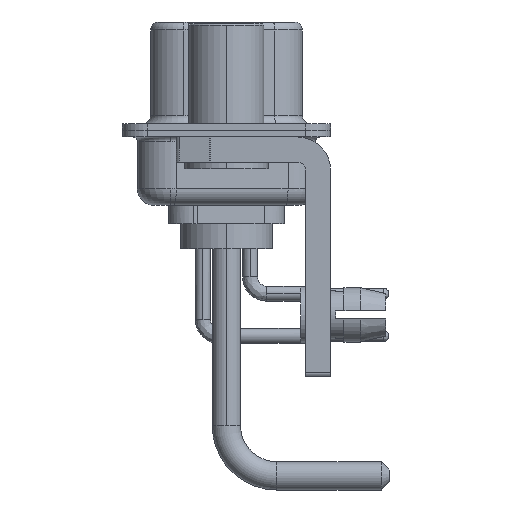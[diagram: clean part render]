
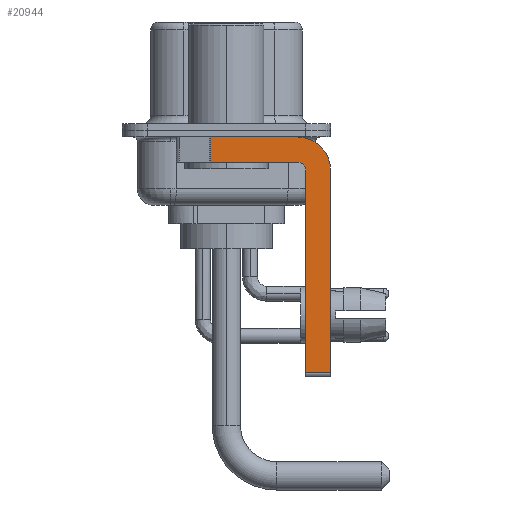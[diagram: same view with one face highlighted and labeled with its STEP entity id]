
A CAD part, left-side view. The second image highlights one B-rep face of the part: STEP entity #20944.
In plain terms, the highlighted planar face has unit normal (-1, 0, 0).
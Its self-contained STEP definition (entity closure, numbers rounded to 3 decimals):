
#20 = DIRECTION ( 'NONE',  ( 0., 0., -1. ) ) ;
#337 = VERTEX_POINT ( 'NONE', #24477 ) ;
#1652 = EDGE_CURVE ( 'NONE', #337, #20494, #12651, .T. ) ;
#2260 = LINE ( 'NONE', #12164, #22588 ) ;
#2328 = VECTOR ( 'NONE', #13168, 1000. ) ;
#2403 = VERTEX_POINT ( 'NONE', #24081 ) ;
#4465 = AXIS2_PLACEMENT_3D ( 'NONE', #7606, #7296, #17183 ) ;
#4870 = VERTEX_POINT ( 'NONE', #11476 ) ;
#5042 = VECTOR ( 'NONE', #24944, 1000. ) ;
#5121 = VERTEX_POINT ( 'NONE', #23053 ) ;
#6582 = CARTESIAN_POINT ( 'NONE',  ( -2.9, -4.25, -1.9 ) ) ;
#6725 = DIRECTION ( 'NONE',  ( 1., 0., 0. ) ) ;
#6737 = VERTEX_POINT ( 'NONE', #23987 ) ;
#6843 = EDGE_CURVE ( 'NONE', #337, #6737, #29660, .T. ) ;
#6912 = DIRECTION ( 'NONE',  ( 0., 1., 0. ) ) ;
#7203 = EDGE_LOOP ( 'NONE', ( #14572, #30391, #12723, #10766, #14267, #25558, #28671, #17697 ) ) ;
#7296 = DIRECTION ( 'NONE',  ( -1., 0., 0. ) ) ;
#7606 = CARTESIAN_POINT ( 'NONE',  ( -2.9, -4.25, -2.4 ) ) ;
#8522 = EDGE_CURVE ( 'NONE', #20494, #2403, #25311, .T. ) ;
#9127 = DIRECTION ( 'NONE',  ( 0., 0., -1. ) ) ;
#9953 = LINE ( 'NONE', #19835, #12711 ) ;
#10766 = ORIENTED_EDGE ( 'NONE', *, *, #31283, .F. ) ;
#11423 = CARTESIAN_POINT ( 'NONE',  ( -2.9, -4.25, -2.4 ) ) ;
#11476 = CARTESIAN_POINT ( 'NONE',  ( -2.9, -4.75, -2.4 ) ) ;
#11678 = EDGE_CURVE ( 'NONE', #5121, #16622, #9953, .T. ) ;
#11955 = EDGE_CURVE ( 'NONE', #2403, #16622, #28383, .T. ) ;
#12164 = CARTESIAN_POINT ( 'NONE',  ( -2.9, -4.75, -14.8 ) ) ;
#12651 = LINE ( 'NONE', #20271, #25658 ) ;
#12711 = VECTOR ( 'NONE', #29723, 1000. ) ;
#12723 = ORIENTED_EDGE ( 'NONE', *, *, #22048, .F. ) ;
#13168 = DIRECTION ( 'NONE',  ( 0., 0., -1. ) ) ;
#13490 = CARTESIAN_POINT ( 'NONE',  ( -2.9, -6.25, -2.4 ) ) ;
#14267 = ORIENTED_EDGE ( 'NONE', *, *, #31288, .F. ) ;
#14572 = ORIENTED_EDGE ( 'NONE', *, *, #1652, .F. ) ;
#15077 = DIRECTION ( 'NONE',  ( 0., 0., 1. ) ) ;
#15804 = FACE_OUTER_BOUND ( 'NONE', #7203, .T. ) ;
#16125 = DIRECTION ( 'NONE',  ( 1., 0., 0. ) ) ;
#16167 = CARTESIAN_POINT ( 'NONE',  ( -2.9, -4.25, -0.4 ) ) ;
#16622 = VERTEX_POINT ( 'NONE', #31142 ) ;
#17183 = DIRECTION ( 'NONE',  ( 0., 0., 1. ) ) ;
#17697 = ORIENTED_EDGE ( 'NONE', *, *, #8522, .F. ) ;
#19469 = CIRCLE ( 'NONE', #4465, 0.5 ) ;
#19767 = VECTOR ( 'NONE', #6912, 1000. ) ;
#19835 = CARTESIAN_POINT ( 'NONE',  ( -2.9, -4.25, -14.55 ) ) ;
#20271 = CARTESIAN_POINT ( 'NONE',  ( -2.9, 3., -0.4 ) ) ;
#20494 = VERTEX_POINT ( 'NONE', #16167 ) ;
#20810 = PLANE ( 'NONE',  #30058 ) ;
#20944 = ADVANCED_FACE ( 'NONE', ( #15804 ), #20810, .F. ) ;
#22048 = EDGE_CURVE ( 'NONE', #22876, #6737, #29131, .T. ) ;
#22588 = VECTOR ( 'NONE', #15077, 1000. ) ;
#22876 = VERTEX_POINT ( 'NONE', #31615 ) ;
#23053 = CARTESIAN_POINT ( 'NONE',  ( -2.9, -4.75, -14.55 ) ) ;
#23987 = CARTESIAN_POINT ( 'NONE',  ( -2.9, 0.978, -1.9 ) ) ;
#24081 = CARTESIAN_POINT ( 'NONE',  ( -2.9, -6.25, -2.4 ) ) ;
#24304 = CARTESIAN_POINT ( 'NONE',  ( -2.9, 0.978, -1.9 ) ) ;
#24477 = CARTESIAN_POINT ( 'NONE',  ( -2.9, 0.978, -0.4 ) ) ;
#24645 = CARTESIAN_POINT ( 'NONE',  ( -2.9, -4.25, -2.4 ) ) ;
#24944 = DIRECTION ( 'NONE',  ( 0., 0., -1. ) ) ;
#25311 = CIRCLE ( 'NONE', #29463, 2. ) ;
#25558 = ORIENTED_EDGE ( 'NONE', *, *, #11678, .T. ) ;
#25658 = VECTOR ( 'NONE', #29835, 1000. ) ;
#28383 = LINE ( 'NONE', #13490, #2328 ) ;
#28671 = ORIENTED_EDGE ( 'NONE', *, *, #11955, .F. ) ;
#29131 = LINE ( 'NONE', #6582, #19767 ) ;
#29463 = AXIS2_PLACEMENT_3D ( 'NONE', #24645, #6725, #20 ) ;
#29660 = LINE ( 'NONE', #24304, #5042 ) ;
#29723 = DIRECTION ( 'NONE',  ( 0., -1., 0. ) ) ;
#29835 = DIRECTION ( 'NONE',  ( 0., -1., 0. ) ) ;
#30058 = AXIS2_PLACEMENT_3D ( 'NONE', #11423, #16125, #9127 ) ;
#30391 = ORIENTED_EDGE ( 'NONE', *, *, #6843, .T. ) ;
#31142 = CARTESIAN_POINT ( 'NONE',  ( -2.9, -6.25, -14.55 ) ) ;
#31283 = EDGE_CURVE ( 'NONE', #4870, #22876, #19469, .T. ) ;
#31288 = EDGE_CURVE ( 'NONE', #5121, #4870, #2260, .T. ) ;
#31615 = CARTESIAN_POINT ( 'NONE',  ( -2.9, -4.25, -1.9 ) ) ;
